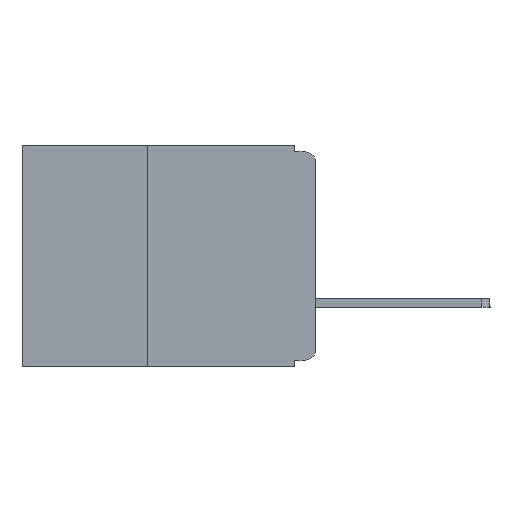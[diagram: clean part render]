
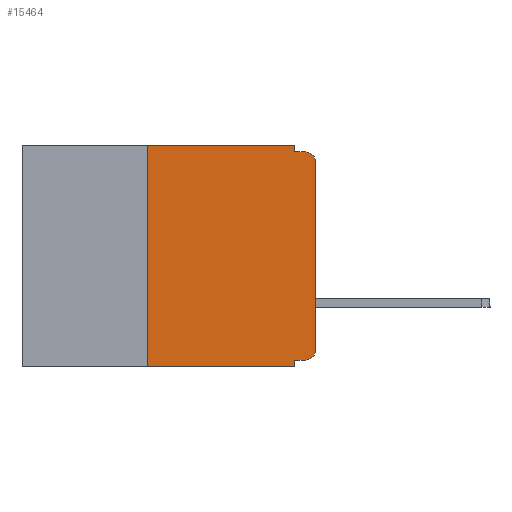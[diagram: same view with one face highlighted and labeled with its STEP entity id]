
A CAD part, left-side view. The second image highlights one B-rep face of the part: STEP entity #15464.
In plain terms, the highlighted planar face has unit normal (-1, 0, 0).
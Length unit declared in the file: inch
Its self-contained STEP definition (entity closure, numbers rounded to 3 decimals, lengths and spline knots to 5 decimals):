
#129 = CARTESIAN_POINT ( 'NONE',  ( 0., 0.031, -0.32 ) ) ;
#217 = CARTESIAN_POINT ( 'NONE',  ( 0., 0.437, 0. ) ) ;
#231 = ORIENTED_EDGE ( 'NONE', *, *, #12007, .F. ) ;
#256 = DIRECTION ( 'NONE',  ( 0., 0., 1. ) ) ;
#620 = DIRECTION ( 'NONE',  ( 0., 0., -1. ) ) ;
#992 = CARTESIAN_POINT ( 'NONE',  ( 0., 0.031, -0.33 ) ) ;
#1414 = CIRCLE ( 'NONE', #18222, 0.015 ) ;
#2128 = DIRECTION ( 'NONE',  ( 0., 0., -1. ) ) ;
#2266 = ORIENTED_EDGE ( 'NONE', *, *, #15653, .F. ) ;
#2328 = VERTEX_POINT ( 'NONE', #992 ) ;
#2339 = EDGE_CURVE ( 'NONE', #3184, #20166, #19507, .T. ) ;
#3184 = VERTEX_POINT ( 'NONE', #21680 ) ;
#3646 = DIRECTION ( 'NONE',  ( 0., 0., 1. ) ) ;
#4127 = VECTOR ( 'NONE', #256, 39.37008 ) ;
#4436 = CARTESIAN_POINT ( 'NONE',  ( 0., 0.015, -0.305 ) ) ;
#4702 = ORIENTED_EDGE ( 'NONE', *, *, #24419, .F. ) ;
#4803 = LINE ( 'NONE', #24696, #13231 ) ;
#6052 = CARTESIAN_POINT ( 'NONE',  ( 0., 0., 0. ) ) ;
#6061 = EDGE_CURVE ( 'NONE', #19632, #2328, #16612, .T. ) ;
#6157 = CARTESIAN_POINT ( 'NONE',  ( 0., 0., -0.01 ) ) ;
#6359 = DIRECTION ( 'NONE',  ( 0., 0., -1. ) ) ;
#6360 = EDGE_CURVE ( 'NONE', #21879, #20324, #19586, .T. ) ;
#6418 = VERTEX_POINT ( 'NONE', #19198 ) ;
#6421 = VECTOR ( 'NONE', #16296, 39.37008 ) ;
#6453 = ORIENTED_EDGE ( 'NONE', *, *, #12829, .F. ) ;
#6498 = VECTOR ( 'NONE', #16156, 39.37008 ) ;
#6594 = ORIENTED_EDGE ( 'NONE', *, *, #6360, .F. ) ;
#6786 = ORIENTED_EDGE ( 'NONE', *, *, #9632, .F. ) ;
#7079 = CARTESIAN_POINT ( 'NONE',  ( 0., 0.437, 0. ) ) ;
#7183 = CARTESIAN_POINT ( 'NONE',  ( 0., 0.031, -0.01 ) ) ;
#7243 = ORIENTED_EDGE ( 'NONE', *, *, #6061, .T. ) ;
#7591 = CARTESIAN_POINT ( 'NONE',  ( 0., 0., -0.32 ) ) ;
#8727 = VECTOR ( 'NONE', #16616, 39.37008 ) ;
#8803 = VECTOR ( 'NONE', #17101, 39.37008 ) ;
#9039 = AXIS2_PLACEMENT_3D ( 'NONE', #12054, #10467, #10416 ) ;
#9126 = CARTESIAN_POINT ( 'NONE',  ( 0., 0.015, -0.01 ) ) ;
#9632 = EDGE_CURVE ( 'NONE', #20324, #2328, #13383, .T. ) ;
#9739 = EDGE_LOOP ( 'NONE', ( #20744, #16848, #231, #2266, #4702, #6453, #7243, #6786, #6594, #22364 ) ) ;
#10000 = DIRECTION ( 'NONE',  ( 0., -1., 0. ) ) ;
#10416 = DIRECTION ( 'NONE',  ( 0., 0., -1. ) ) ;
#10467 = DIRECTION ( 'NONE',  ( -1., 0., 0. ) ) ;
#11181 = CARTESIAN_POINT ( 'NONE',  ( 0., 0.25, 0. ) ) ;
#11320 = FACE_OUTER_BOUND ( 'NONE', #9739, .T. ) ;
#11667 = PLANE ( 'NONE',  #12769 ) ;
#12007 = EDGE_CURVE ( 'NONE', #23840, #20166, #17136, .T. ) ;
#12054 = CARTESIAN_POINT ( 'NONE',  ( 0., 0.015, -0.025 ) ) ;
#12200 = VECTOR ( 'NONE', #620, 39.37008 ) ;
#12250 = LINE ( 'NONE', #14261, #6498 ) ;
#12769 = AXIS2_PLACEMENT_3D ( 'NONE', #217, #13611, #2128 ) ;
#12829 = EDGE_CURVE ( 'NONE', #19632, #19611, #4803, .T. ) ;
#13231 = VECTOR ( 'NONE', #3646, 39.37008 ) ;
#13359 = CARTESIAN_POINT ( 'NONE',  ( 0., 0., -0.305 ) ) ;
#13383 = LINE ( 'NONE', #23555, #12200 ) ;
#13611 = DIRECTION ( 'NONE',  ( 1., 0., 0. ) ) ;
#14261 = CARTESIAN_POINT ( 'NONE',  ( 0., 0.031, 0. ) ) ;
#14908 = EDGE_CURVE ( 'NONE', #20266, #3184, #14937, .T. ) ;
#14937 = LINE ( 'NONE', #6052, #4127 ) ;
#15464 = ADVANCED_FACE ( 'NONE', ( #11320 ), #11667, .F. ) ;
#15653 = EDGE_CURVE ( 'NONE', #6418, #23840, #12250, .T. ) ;
#16156 = DIRECTION ( 'NONE',  ( 0., 0., -1. ) ) ;
#16296 = DIRECTION ( 'NONE',  ( 0., -1., 0. ) ) ;
#16546 = VECTOR ( 'NONE', #10000, 39.37008 ) ;
#16612 = LINE ( 'NONE', #23932, #6421 ) ;
#16616 = DIRECTION ( 'NONE',  ( 0., -1., 0. ) ) ;
#16848 = ORIENTED_EDGE ( 'NONE', *, *, #2339, .T. ) ;
#17101 = DIRECTION ( 'NONE',  ( 0., 1., 0. ) ) ;
#17136 = LINE ( 'NONE', #6157, #16546 ) ;
#17852 = DIRECTION ( 'NONE',  ( -1., 0., 0. ) ) ;
#18222 = AXIS2_PLACEMENT_3D ( 'NONE', #4436, #17852, #6359 ) ;
#19198 = CARTESIAN_POINT ( 'NONE',  ( 0., 0.031, 0. ) ) ;
#19507 = CIRCLE ( 'NONE', #9039, 0.015 ) ;
#19586 = LINE ( 'NONE', #7591, #8803 ) ;
#19611 = VERTEX_POINT ( 'NONE', #11181 ) ;
#19632 = VERTEX_POINT ( 'NONE', #24599 ) ;
#20166 = VERTEX_POINT ( 'NONE', #9126 ) ;
#20266 = VERTEX_POINT ( 'NONE', #13359 ) ;
#20324 = VERTEX_POINT ( 'NONE', #129 ) ;
#20744 = ORIENTED_EDGE ( 'NONE', *, *, #14908, .T. ) ;
#21448 = EDGE_CURVE ( 'NONE', #21879, #20266, #1414, .T. ) ;
#21680 = CARTESIAN_POINT ( 'NONE',  ( 0., 0., -0.025 ) ) ;
#21879 = VERTEX_POINT ( 'NONE', #22961 ) ;
#22364 = ORIENTED_EDGE ( 'NONE', *, *, #21448, .T. ) ;
#22961 = CARTESIAN_POINT ( 'NONE',  ( 0., 0.015, -0.32 ) ) ;
#23555 = CARTESIAN_POINT ( 'NONE',  ( 0., 0.031, -0.33 ) ) ;
#23840 = VERTEX_POINT ( 'NONE', #7183 ) ;
#23932 = CARTESIAN_POINT ( 'NONE',  ( 0., 0.437, -0.33 ) ) ;
#24022 = LINE ( 'NONE', #7079, #8727 ) ;
#24419 = EDGE_CURVE ( 'NONE', #19611, #6418, #24022, .T. ) ;
#24599 = CARTESIAN_POINT ( 'NONE',  ( 0., 0.25, -0.33 ) ) ;
#24696 = CARTESIAN_POINT ( 'NONE',  ( 0., 0.25, -0.33 ) ) ;
